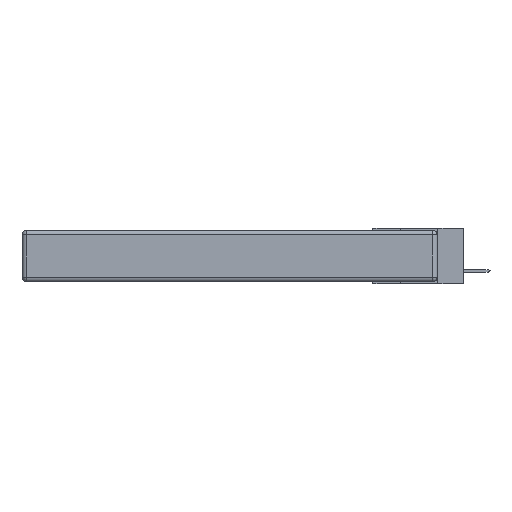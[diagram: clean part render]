
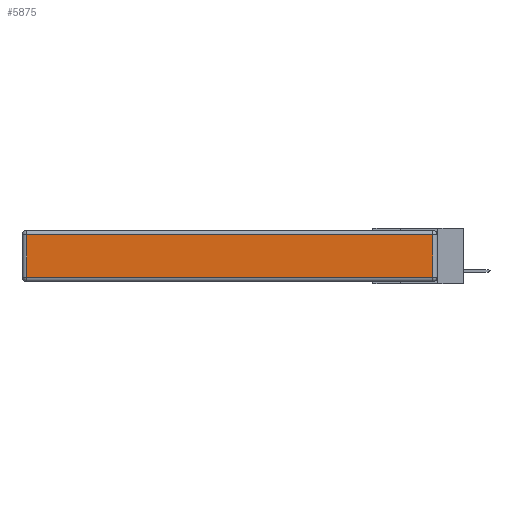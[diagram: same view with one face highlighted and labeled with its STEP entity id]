
A CAD part, left-side view. The second image highlights one B-rep face of the part: STEP entity #5875.
In plain terms, the highlighted planar face has unit normal (-1, 0, 0).
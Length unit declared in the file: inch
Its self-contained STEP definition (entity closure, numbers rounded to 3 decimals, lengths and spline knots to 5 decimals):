
#599 = CARTESIAN_POINT ( 'NONE',  ( 0., 2.72, -0.03 ) ) ;
#1018 = VERTEX_POINT ( 'NONE', #12642 ) ;
#1299 = CARTESIAN_POINT ( 'NONE',  ( 0., 0.03, -0.03 ) ) ;
#4649 = EDGE_CURVE ( 'NONE', #1018, #12615, #8015, .T. ) ;
#4676 = EDGE_CURVE ( 'NONE', #12615, #22478, #21886, .T. ) ;
#5232 = CARTESIAN_POINT ( 'NONE',  ( 0., 0.03, -0.343 ) ) ;
#5875 = ADVANCED_FACE ( 'NONE', ( #10135 ), #21491, .T. ) ;
#6196 = ORIENTED_EDGE ( 'NONE', *, *, #4676, .T. ) ;
#6898 = ORIENTED_EDGE ( 'NONE', *, *, #11555, .T. ) ;
#8015 = LINE ( 'NONE', #5232, #11025 ) ;
#8420 = VECTOR ( 'NONE', #20758, 39.37008 ) ;
#8578 = DIRECTION ( 'NONE',  ( 0., 1., 0. ) ) ;
#9591 = ORIENTED_EDGE ( 'NONE', *, *, #14891, .T. ) ;
#10135 = FACE_OUTER_BOUND ( 'NONE', #18498, .T. ) ;
#11025 = VECTOR ( 'NONE', #18885, 39.37008 ) ;
#11090 = DIRECTION ( 'NONE',  ( -1., 0., 0. ) ) ;
#11555 = EDGE_CURVE ( 'NONE', #12277, #1018, #13500, .T. ) ;
#11922 = CARTESIAN_POINT ( 'NONE',  ( 0., 2.75, -0.03 ) ) ;
#12146 = DIRECTION ( 'NONE',  ( 0., -1., 0. ) ) ;
#12277 = VERTEX_POINT ( 'NONE', #21153 ) ;
#12310 = CARTESIAN_POINT ( 'NONE',  ( 0., 0., -0.313 ) ) ;
#12615 = VERTEX_POINT ( 'NONE', #1299 ) ;
#12642 = CARTESIAN_POINT ( 'NONE',  ( 0., 0.03, -0.313 ) ) ;
#12658 = VECTOR ( 'NONE', #8578, 39.37008 ) ;
#13500 = LINE ( 'NONE', #12310, #16467 ) ;
#14467 = CARTESIAN_POINT ( 'NONE',  ( 0., 0., -0.343 ) ) ;
#14891 = EDGE_CURVE ( 'NONE', #22478, #12277, #20358, .T. ) ;
#16467 = VECTOR ( 'NONE', #12146, 39.37008 ) ;
#17203 = CARTESIAN_POINT ( 'NONE',  ( 0., 2.72, -0.343 ) ) ;
#18180 = ORIENTED_EDGE ( 'NONE', *, *, #4649, .T. ) ;
#18498 = EDGE_LOOP ( 'NONE', ( #6898, #18180, #6196, #9591 ) ) ;
#18885 = DIRECTION ( 'NONE',  ( 0., 0., 1. ) ) ;
#19384 = AXIS2_PLACEMENT_3D ( 'NONE', #14467, #11090, #21266 ) ;
#20358 = LINE ( 'NONE', #17203, #8420 ) ;
#20758 = DIRECTION ( 'NONE',  ( 0., 0., -1. ) ) ;
#21153 = CARTESIAN_POINT ( 'NONE',  ( 0., 2.72, -0.313 ) ) ;
#21266 = DIRECTION ( 'NONE',  ( 0., 0., 1. ) ) ;
#21491 = PLANE ( 'NONE',  #19384 ) ;
#21886 = LINE ( 'NONE', #11922, #12658 ) ;
#22478 = VERTEX_POINT ( 'NONE', #599 ) ;
